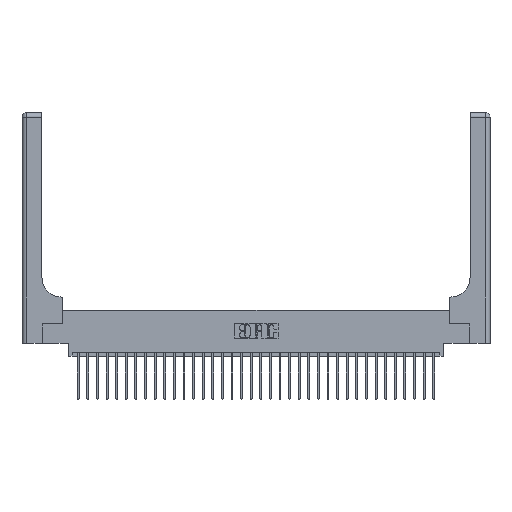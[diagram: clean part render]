
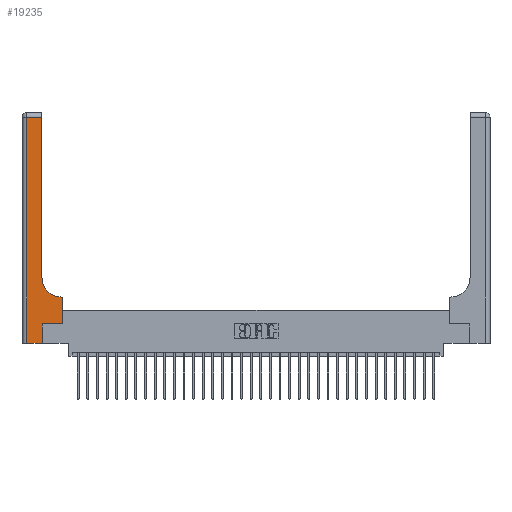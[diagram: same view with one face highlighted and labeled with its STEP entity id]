
A CAD part, top view. The second image highlights one B-rep face of the part: STEP entity #19235.
In plain terms, the highlighted planar face has unit normal (0, 0, 1).
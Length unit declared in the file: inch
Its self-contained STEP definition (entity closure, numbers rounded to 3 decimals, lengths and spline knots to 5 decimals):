
#146 = LINE ( 'NONE', #8381, #24651 ) ;
#817 = CIRCLE ( 'NONE', #13914, 0.25 ) ;
#1032 = CARTESIAN_POINT ( 'NONE',  ( 0.265, 0., 0.37 ) ) ;
#1040 = ORIENTED_EDGE ( 'NONE', *, *, #19929, .T. ) ;
#1212 = DIRECTION ( 'NONE',  ( 0., 0., -1. ) ) ;
#1419 = VECTOR ( 'NONE', #30383, 39.37008 ) ;
#1664 = CARTESIAN_POINT ( 'NONE',  ( 0.528, 0.6, 0.37 ) ) ;
#2474 = CARTESIAN_POINT ( 'NONE',  ( 0.26, 3., 0.37 ) ) ;
#2719 = CARTESIAN_POINT ( 'NONE',  ( 0., 0., 0.37 ) ) ;
#2811 = DIRECTION ( 'NONE',  ( 1., 0., 0. ) ) ;
#3168 = ORIENTED_EDGE ( 'NONE', *, *, #4228, .T. ) ;
#3718 = EDGE_CURVE ( 'NONE', #23747, #8444, #30522, .T. ) ;
#3854 = EDGE_CURVE ( 'NONE', #20238, #22366, #20545, .T. ) ;
#4228 = EDGE_CURVE ( 'NONE', #4904, #20238, #13124, .T. ) ;
#4898 = DIRECTION ( 'NONE',  ( 0., 1., 0. ) ) ;
#4904 = VERTEX_POINT ( 'NONE', #19481 ) ;
#5138 = DIRECTION ( 'NONE',  ( 1., 0., 0. ) ) ;
#6949 = VECTOR ( 'NONE', #10610, 39.37008 ) ;
#6969 = EDGE_LOOP ( 'NONE', ( #16527, #1040, #13840, #15195, #23458, #3168, #14079, #10815, #16493 ) ) ;
#7344 = EDGE_CURVE ( 'NONE', #22366, #8123, #14087, .T. ) ;
#7388 = CARTESIAN_POINT ( 'NONE',  ( 0.26, 2.94, 0.37 ) ) ;
#7551 = VERTEX_POINT ( 'NONE', #7388 ) ;
#8007 = DIRECTION ( 'NONE',  ( 0., 0., -1. ) ) ;
#8095 = CARTESIAN_POINT ( 'NONE',  ( 0.06, 2.94, 0.37 ) ) ;
#8123 = VERTEX_POINT ( 'NONE', #9679 ) ;
#8369 = CARTESIAN_POINT ( 'NONE',  ( 0.528, 0.25, 0.37 ) ) ;
#8381 = CARTESIAN_POINT ( 'NONE',  ( 0., 2.94, 0.37 ) ) ;
#8444 = VERTEX_POINT ( 'NONE', #1032 ) ;
#8690 = VECTOR ( 'NONE', #24911, 39.37008 ) ;
#9340 = CARTESIAN_POINT ( 'NONE',  ( 0.265, 0., 0.37 ) ) ;
#9679 = CARTESIAN_POINT ( 'NONE',  ( 0.51, 0.6, 0.37 ) ) ;
#9779 = CARTESIAN_POINT ( 'NONE',  ( 0.26, 0.85, 0.37 ) ) ;
#9976 = LINE ( 'NONE', #9340, #15524 ) ;
#10610 = DIRECTION ( 'NONE',  ( 0., -1., 0. ) ) ;
#10815 = ORIENTED_EDGE ( 'NONE', *, *, #7344, .T. ) ;
#13124 = LINE ( 'NONE', #14673, #18659 ) ;
#13840 = ORIENTED_EDGE ( 'NONE', *, *, #14224, .T. ) ;
#13914 = AXIS2_PLACEMENT_3D ( 'NONE', #22192, #8007, #24564 ) ;
#14079 = ORIENTED_EDGE ( 'NONE', *, *, #3854, .T. ) ;
#14087 = LINE ( 'NONE', #16255, #1419 ) ;
#14224 = EDGE_CURVE ( 'NONE', #17343, #23747, #19566, .T. ) ;
#14673 = CARTESIAN_POINT ( 'NONE',  ( 0.265, 0.25, 0.37 ) ) ;
#15195 = ORIENTED_EDGE ( 'NONE', *, *, #3718, .T. ) ;
#15475 = PLANE ( 'NONE',  #19096 ) ;
#15524 = VECTOR ( 'NONE', #30638, 39.37008 ) ;
#16255 = CARTESIAN_POINT ( 'NONE',  ( 0.26, 0.6, 0.37 ) ) ;
#16493 = ORIENTED_EDGE ( 'NONE', *, *, #22782, .T. ) ;
#16527 = ORIENTED_EDGE ( 'NONE', *, *, #29933, .T. ) ;
#16745 = VECTOR ( 'NONE', #4898, 39.37008 ) ;
#17343 = VERTEX_POINT ( 'NONE', #8095 ) ;
#17577 = EDGE_CURVE ( 'NONE', #8444, #4904, #9976, .T. ) ;
#17728 = CARTESIAN_POINT ( 'NONE',  ( 0., 3., 0.37 ) ) ;
#17831 = DIRECTION ( 'NONE',  ( -1., 0., 0. ) ) ;
#17951 = VECTOR ( 'NONE', #5138, 39.37008 ) ;
#18659 = VECTOR ( 'NONE', #2811, 39.37008 ) ;
#19096 = AXIS2_PLACEMENT_3D ( 'NONE', #17728, #1212, #17831 ) ;
#19235 = ADVANCED_FACE ( 'NONE', ( #22804 ), #15475, .F. ) ;
#19481 = CARTESIAN_POINT ( 'NONE',  ( 0.265, 0.25, 0.37 ) ) ;
#19566 = LINE ( 'NONE', #27116, #6949 ) ;
#19661 = CARTESIAN_POINT ( 'NONE',  ( 0.06, 0., 0.37 ) ) ;
#19929 = EDGE_CURVE ( 'NONE', #7551, #17343, #146, .T. ) ;
#20238 = VERTEX_POINT ( 'NONE', #26868 ) ;
#20545 = LINE ( 'NONE', #8369, #8690 ) ;
#22192 = CARTESIAN_POINT ( 'NONE',  ( 0.51, 0.85, 0.37 ) ) ;
#22366 = VERTEX_POINT ( 'NONE', #1664 ) ;
#22782 = EDGE_CURVE ( 'NONE', #8123, #26271, #817, .T. ) ;
#22804 = FACE_OUTER_BOUND ( 'NONE', #6969, .T. ) ;
#23458 = ORIENTED_EDGE ( 'NONE', *, *, #17577, .T. ) ;
#23747 = VERTEX_POINT ( 'NONE', #19661 ) ;
#24564 = DIRECTION ( 'NONE',  ( 1., 0., 0. ) ) ;
#24651 = VECTOR ( 'NONE', #24929, 39.37008 ) ;
#24911 = DIRECTION ( 'NONE',  ( 0., 1., 0. ) ) ;
#24929 = DIRECTION ( 'NONE',  ( -1., 0., 0. ) ) ;
#26271 = VERTEX_POINT ( 'NONE', #9779 ) ;
#26868 = CARTESIAN_POINT ( 'NONE',  ( 0.528, 0.25, 0.37 ) ) ;
#27116 = CARTESIAN_POINT ( 'NONE',  ( 0.06, 3., 0.37 ) ) ;
#29289 = LINE ( 'NONE', #2474, #16745 ) ;
#29933 = EDGE_CURVE ( 'NONE', #26271, #7551, #29289, .T. ) ;
#30383 = DIRECTION ( 'NONE',  ( -1., 0., 0. ) ) ;
#30522 = LINE ( 'NONE', #2719, #17951 ) ;
#30638 = DIRECTION ( 'NONE',  ( 0., 1., 0. ) ) ;
